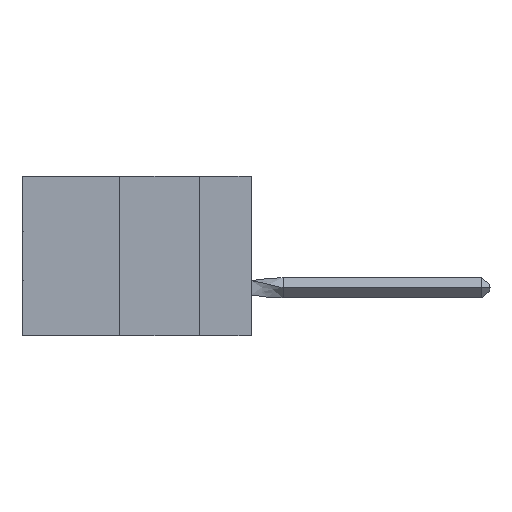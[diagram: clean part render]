
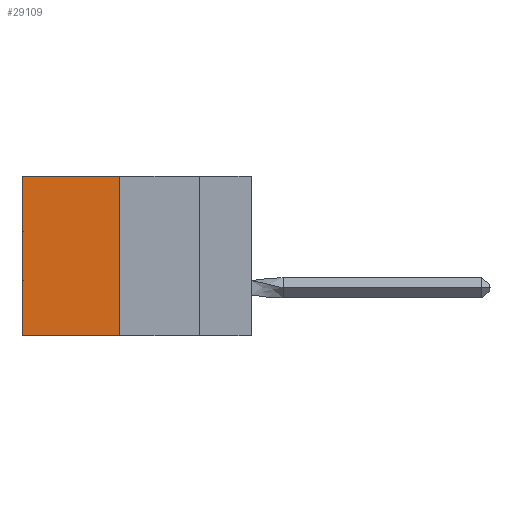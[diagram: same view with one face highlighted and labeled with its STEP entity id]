
A CAD part, left-side view. The second image highlights one B-rep face of the part: STEP entity #29109.
In plain terms, the highlighted planar face has unit normal (-1, 0, 0).
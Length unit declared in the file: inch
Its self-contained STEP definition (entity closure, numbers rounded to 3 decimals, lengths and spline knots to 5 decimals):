
#1598 = LINE ( 'NONE', #22807, #10618 ) ;
#2105 = CARTESIAN_POINT ( 'NONE',  ( 0.305, 0.413, -0.5 ) ) ;
#4421 = AXIS2_PLACEMENT_3D ( 'NONE', #42273, #43501, #7270 ) ;
#5692 = DIRECTION ( 'NONE',  ( 0., 0., -1. ) ) ;
#7221 = EDGE_LOOP ( 'NONE', ( #27630, #43158, #39481, #34352 ) ) ;
#7270 = DIRECTION ( 'NONE',  ( 0., 0., -1. ) ) ;
#7895 = CARTESIAN_POINT ( 'NONE',  ( 0.305, 0.413, 0. ) ) ;
#10618 = VECTOR ( 'NONE', #19186, 39.37008 ) ;
#12745 = CARTESIAN_POINT ( 'NONE',  ( 0.305, 0.72, 0. ) ) ;
#13336 = EDGE_CURVE ( 'NONE', #15272, #26762, #17323, .T. ) ;
#14602 = EDGE_CURVE ( 'NONE', #15272, #31811, #41488, .T. ) ;
#14918 = EDGE_CURVE ( 'NONE', #26762, #26807, #16246, .T. ) ;
#15272 = VERTEX_POINT ( 'NONE', #7895 ) ;
#16246 = LINE ( 'NONE', #39608, #32609 ) ;
#17323 = LINE ( 'NONE', #2105, #25230 ) ;
#19186 = DIRECTION ( 'NONE',  ( 0., 0., -1. ) ) ;
#21942 = CARTESIAN_POINT ( 'NONE',  ( 0.305, 0.72, -0.5 ) ) ;
#22807 = CARTESIAN_POINT ( 'NONE',  ( 0.305, 0.72, -0.5 ) ) ;
#23311 = FACE_OUTER_BOUND ( 'NONE', #7221, .T. ) ;
#23319 = DIRECTION ( 'NONE',  ( 0., 1., 0. ) ) ;
#24934 = CARTESIAN_POINT ( 'NONE',  ( 0.305, 0.413, -0.5 ) ) ;
#25230 = VECTOR ( 'NONE', #5692, 39.37008 ) ;
#26762 = VERTEX_POINT ( 'NONE', #24934 ) ;
#26807 = VERTEX_POINT ( 'NONE', #21942 ) ;
#27630 = ORIENTED_EDGE ( 'NONE', *, *, #35647, .T. ) ;
#29109 = ADVANCED_FACE ( 'NONE', ( #23311 ), #38530, .F. ) ;
#31811 = VERTEX_POINT ( 'NONE', #12745 ) ;
#31861 = VECTOR ( 'NONE', #23319, 39.37008 ) ;
#32609 = VECTOR ( 'NONE', #35633, 39.37008 ) ;
#34352 = ORIENTED_EDGE ( 'NONE', *, *, #14602, .T. ) ;
#35633 = DIRECTION ( 'NONE',  ( 0., 1., 0. ) ) ;
#35647 = EDGE_CURVE ( 'NONE', #31811, #26807, #1598, .T. ) ;
#38530 = PLANE ( 'NONE',  #4421 ) ;
#39481 = ORIENTED_EDGE ( 'NONE', *, *, #13336, .F. ) ;
#39608 = CARTESIAN_POINT ( 'NONE',  ( 0.305, 0.413, -0.5 ) ) ;
#41488 = LINE ( 'NONE', #44750, #31861 ) ;
#42273 = CARTESIAN_POINT ( 'NONE',  ( 0.305, 0.413, -0.5 ) ) ;
#43158 = ORIENTED_EDGE ( 'NONE', *, *, #14918, .F. ) ;
#43501 = DIRECTION ( 'NONE',  ( 1., 0., 0. ) ) ;
#44750 = CARTESIAN_POINT ( 'NONE',  ( 0.305, 0.413, 0. ) ) ;
